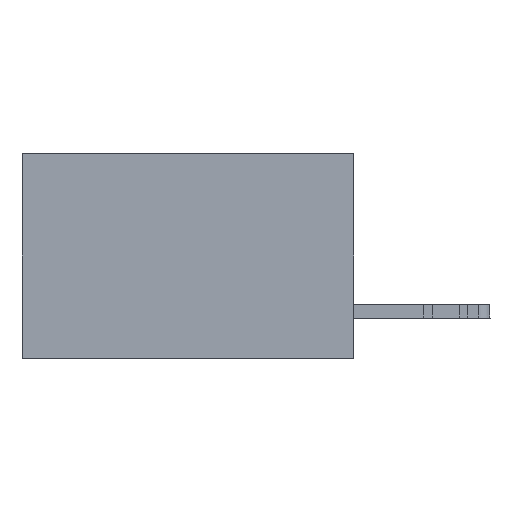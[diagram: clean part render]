
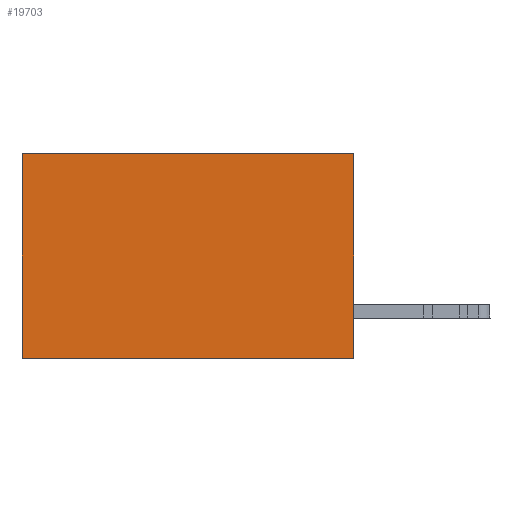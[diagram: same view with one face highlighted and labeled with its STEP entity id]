
A CAD part, left-side view. The second image highlights one B-rep face of the part: STEP entity #19703.
In plain terms, the highlighted planar face has unit normal (-1, 0, 0).
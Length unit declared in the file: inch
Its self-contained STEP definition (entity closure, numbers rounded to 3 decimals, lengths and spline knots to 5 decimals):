
#3262 = VECTOR ( 'NONE', #33599, 39.37008 ) ;
#5599 = CARTESIAN_POINT ( 'NONE',  ( 0.2875, 0., 0. ) ) ;
#7188 = CARTESIAN_POINT ( 'NONE',  ( 0.2875, 0., 0. ) ) ;
#8753 = FACE_OUTER_BOUND ( 'NONE', #33393, .T. ) ;
#9324 = DIRECTION ( 'NONE',  ( 0., 0., -1. ) ) ;
#9891 = VECTOR ( 'NONE', #41248, 39.37008 ) ;
#13015 = EDGE_CURVE ( 'NONE', #18093, #20715, #28424, .T. ) ;
#13989 = VERTEX_POINT ( 'NONE', #14780 ) ;
#14037 = VECTOR ( 'NONE', #35788, 39.37008 ) ;
#14780 = CARTESIAN_POINT ( 'NONE',  ( 0.2875, 0., -0.37 ) ) ;
#17226 = EDGE_CURVE ( 'NONE', #18093, #13989, #46690, .T. ) ;
#17543 = PLANE ( 'NONE',  #18325 ) ;
#17959 = CARTESIAN_POINT ( 'NONE',  ( 0.2875, 0.6, -0.37 ) ) ;
#18093 = VERTEX_POINT ( 'NONE', #7188 ) ;
#18325 = AXIS2_PLACEMENT_3D ( 'NONE', #5599, #24298, #26930 ) ;
#18830 = ORIENTED_EDGE ( 'NONE', *, *, #41641, .T. ) ;
#19703 = ADVANCED_FACE ( 'NONE', ( #8753 ), #17543, .F. ) ;
#20414 = ORIENTED_EDGE ( 'NONE', *, *, #13015, .T. ) ;
#20715 = VERTEX_POINT ( 'NONE', #31473 ) ;
#24298 = DIRECTION ( 'NONE',  ( 1., 0., 0. ) ) ;
#25007 = EDGE_CURVE ( 'NONE', #13989, #38826, #27861, .T. ) ;
#26930 = DIRECTION ( 'NONE',  ( 0., 0., -1. ) ) ;
#27861 = LINE ( 'NONE', #48854, #9891 ) ;
#28424 = LINE ( 'NONE', #29745, #3262 ) ;
#29745 = CARTESIAN_POINT ( 'NONE',  ( 0.2875, 0., 0. ) ) ;
#31367 = CARTESIAN_POINT ( 'NONE',  ( 0.2875, 0.6, 0. ) ) ;
#31473 = CARTESIAN_POINT ( 'NONE',  ( 0.2875, 0.6, 0. ) ) ;
#33280 = ORIENTED_EDGE ( 'NONE', *, *, #17226, .F. ) ;
#33393 = EDGE_LOOP ( 'NONE', ( #18830, #44706, #33280, #20414 ) ) ;
#33599 = DIRECTION ( 'NONE',  ( 0., 1., 0. ) ) ;
#35788 = DIRECTION ( 'NONE',  ( 0., 0., -1. ) ) ;
#38826 = VERTEX_POINT ( 'NONE', #17959 ) ;
#41248 = DIRECTION ( 'NONE',  ( 0., 1., 0. ) ) ;
#41641 = EDGE_CURVE ( 'NONE', #20715, #38826, #49593, .T. ) ;
#44706 = ORIENTED_EDGE ( 'NONE', *, *, #25007, .F. ) ;
#46690 = LINE ( 'NONE', #46712, #48557 ) ;
#46712 = CARTESIAN_POINT ( 'NONE',  ( 0.2875, 0., 0. ) ) ;
#48557 = VECTOR ( 'NONE', #9324, 39.37008 ) ;
#48854 = CARTESIAN_POINT ( 'NONE',  ( 0.2875, 0., -0.37 ) ) ;
#49593 = LINE ( 'NONE', #31367, #14037 ) ;
